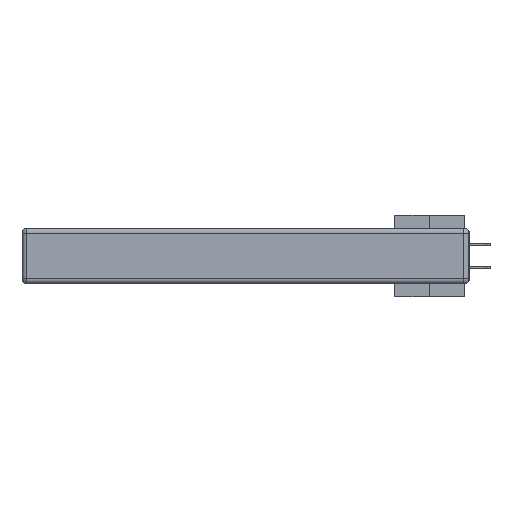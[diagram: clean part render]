
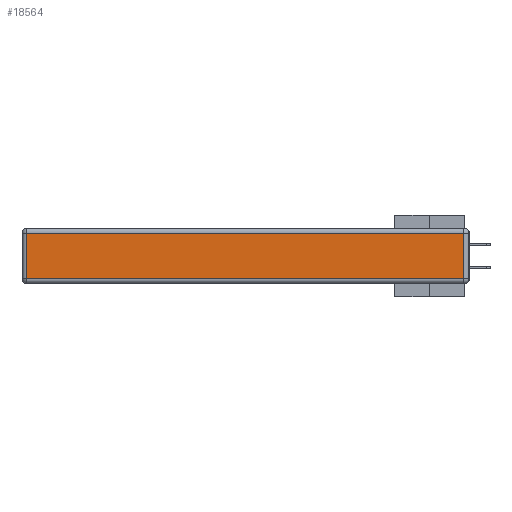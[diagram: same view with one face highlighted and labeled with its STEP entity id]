
A CAD part, left-side view. The second image highlights one B-rep face of the part: STEP entity #18564.
In plain terms, the highlighted planar face has unit normal (-1, 0, 0).
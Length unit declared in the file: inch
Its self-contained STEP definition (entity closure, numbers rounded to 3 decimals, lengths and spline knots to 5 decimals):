
#63 = PLANE ( 'NONE',  #22898 ) ;
#815 = VERTEX_POINT ( 'NONE', #24369 ) ;
#1216 = EDGE_LOOP ( 'NONE', ( #33344, #5694, #17866, #20010 ) ) ;
#1362 = EDGE_CURVE ( 'NONE', #25448, #815, #33154, .T. ) ;
#1833 = DIRECTION ( 'NONE',  ( 0., 1., 0. ) ) ;
#4913 = CARTESIAN_POINT ( 'NONE',  ( 0., 2.72, -0.03 ) ) ;
#5694 = ORIENTED_EDGE ( 'NONE', *, *, #1362, .T. ) ;
#6366 = FACE_OUTER_BOUND ( 'NONE', #1216, .T. ) ;
#6553 = LINE ( 'NONE', #21546, #21915 ) ;
#7891 = LINE ( 'NONE', #16042, #27377 ) ;
#8330 = CARTESIAN_POINT ( 'NONE',  ( 0., 2.72, -0.343 ) ) ;
#12866 = DIRECTION ( 'NONE',  ( 0., 0., 1. ) ) ;
#13319 = DIRECTION ( 'NONE',  ( -1., 0., 0. ) ) ;
#15639 = CARTESIAN_POINT ( 'NONE',  ( 0., 2.72, -0.313 ) ) ;
#16042 = CARTESIAN_POINT ( 'NONE',  ( 0., 0., -0.313 ) ) ;
#16710 = CARTESIAN_POINT ( 'NONE',  ( 0., 0., -0.343 ) ) ;
#17260 = CARTESIAN_POINT ( 'NONE',  ( 0., 0.03, -0.313 ) ) ;
#17866 = ORIENTED_EDGE ( 'NONE', *, *, #23653, .T. ) ;
#18564 = ADVANCED_FACE ( 'NONE', ( #6366 ), #63, .T. ) ;
#19442 = DIRECTION ( 'NONE',  ( 0., 0., 1. ) ) ;
#20010 = ORIENTED_EDGE ( 'NONE', *, *, #28702, .T. ) ;
#20134 = VERTEX_POINT ( 'NONE', #15639 ) ;
#21546 = CARTESIAN_POINT ( 'NONE',  ( 0., 2.75, -0.03 ) ) ;
#21915 = VECTOR ( 'NONE', #1833, 39.37008 ) ;
#22898 = AXIS2_PLACEMENT_3D ( 'NONE', #16710, #13319, #12866 ) ;
#23653 = EDGE_CURVE ( 'NONE', #815, #38732, #6553, .T. ) ;
#24369 = CARTESIAN_POINT ( 'NONE',  ( 0., 0.03, -0.03 ) ) ;
#25381 = DIRECTION ( 'NONE',  ( 0., -1., 0. ) ) ;
#25448 = VERTEX_POINT ( 'NONE', #17260 ) ;
#27377 = VECTOR ( 'NONE', #25381, 39.37008 ) ;
#28702 = EDGE_CURVE ( 'NONE', #38732, #20134, #34037, .T. ) ;
#29408 = VECTOR ( 'NONE', #31383, 39.37008 ) ;
#31383 = DIRECTION ( 'NONE',  ( 0., 0., -1. ) ) ;
#33154 = LINE ( 'NONE', #36339, #39860 ) ;
#33344 = ORIENTED_EDGE ( 'NONE', *, *, #40968, .T. ) ;
#34037 = LINE ( 'NONE', #8330, #29408 ) ;
#36339 = CARTESIAN_POINT ( 'NONE',  ( 0., 0.03, -0.343 ) ) ;
#38732 = VERTEX_POINT ( 'NONE', #4913 ) ;
#39860 = VECTOR ( 'NONE', #19442, 39.37008 ) ;
#40968 = EDGE_CURVE ( 'NONE', #20134, #25448, #7891, .T. ) ;
